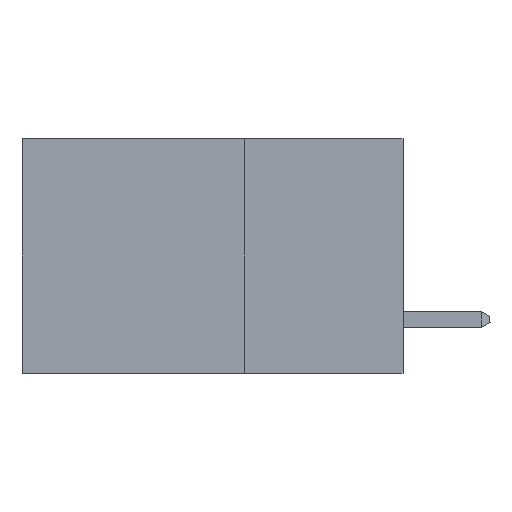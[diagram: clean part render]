
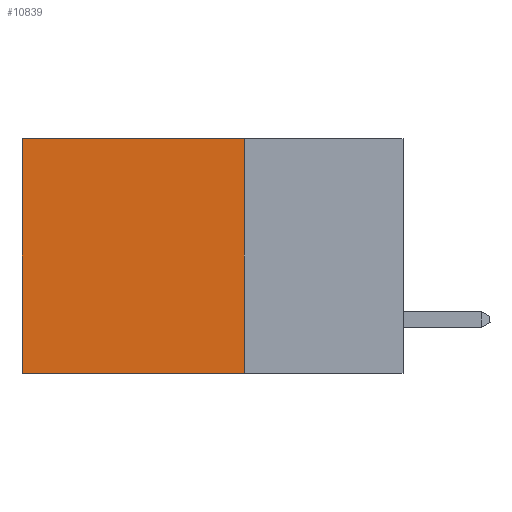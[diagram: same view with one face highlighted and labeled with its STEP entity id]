
A CAD part, left-side view. The second image highlights one B-rep face of the part: STEP entity #10839.
In plain terms, the highlighted planar face has unit normal (-1, 0, 0).
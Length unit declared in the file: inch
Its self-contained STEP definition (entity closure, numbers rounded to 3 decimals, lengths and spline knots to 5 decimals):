
#232 = CARTESIAN_POINT ( 'NONE',  ( 0.2875, 0.25, 0. ) ) ;
#489 = ORIENTED_EDGE ( 'NONE', *, *, #2428, .T. ) ;
#864 = VECTOR ( 'NONE', #17393, 39.37008 ) ;
#1470 = ORIENTED_EDGE ( 'NONE', *, *, #23373, .F. ) ;
#1630 = VERTEX_POINT ( 'NONE', #36720 ) ;
#2127 = VECTOR ( 'NONE', #3511, 39.37008 ) ;
#2197 = LINE ( 'NONE', #10476, #6208 ) ;
#2428 = EDGE_CURVE ( 'NONE', #10773, #30588, #11202, .T. ) ;
#2850 = DIRECTION ( 'NONE',  ( 0., 0., -1. ) ) ;
#3511 = DIRECTION ( 'NONE',  ( 0., 1., 0. ) ) ;
#6208 = VECTOR ( 'NONE', #19549, 39.37008 ) ;
#8319 = EDGE_CURVE ( 'NONE', #30588, #23445, #21845, .T. ) ;
#9410 = CARTESIAN_POINT ( 'NONE',  ( 0.2875, 0.6, -0.37 ) ) ;
#10476 = CARTESIAN_POINT ( 'NONE',  ( 0.2875, 0.25, 0. ) ) ;
#10515 = EDGE_LOOP ( 'NONE', ( #23994, #1470, #16117, #489 ) ) ;
#10773 = VERTEX_POINT ( 'NONE', #232 ) ;
#10839 = ADVANCED_FACE ( 'NONE', ( #13617 ), #36881, .F. ) ;
#11202 = LINE ( 'NONE', #35034, #864 ) ;
#13617 = FACE_OUTER_BOUND ( 'NONE', #10515, .T. ) ;
#16117 = ORIENTED_EDGE ( 'NONE', *, *, #21582, .F. ) ;
#17393 = DIRECTION ( 'NONE',  ( 0., 1., 0. ) ) ;
#18288 = CARTESIAN_POINT ( 'NONE',  ( 0.2875, 0.6, 0. ) ) ;
#19463 = CARTESIAN_POINT ( 'NONE',  ( 0.2875, 0.6, 0. ) ) ;
#19549 = DIRECTION ( 'NONE',  ( 0., 0., -1. ) ) ;
#21582 = EDGE_CURVE ( 'NONE', #10773, #1630, #2197, .T. ) ;
#21845 = LINE ( 'NONE', #19463, #24128 ) ;
#21852 = AXIS2_PLACEMENT_3D ( 'NONE', #31294, #37135, #2850 ) ;
#23373 = EDGE_CURVE ( 'NONE', #1630, #23445, #25505, .T. ) ;
#23445 = VERTEX_POINT ( 'NONE', #9410 ) ;
#23994 = ORIENTED_EDGE ( 'NONE', *, *, #8319, .T. ) ;
#24128 = VECTOR ( 'NONE', #36541, 39.37008 ) ;
#25505 = LINE ( 'NONE', #29323, #2127 ) ;
#29323 = CARTESIAN_POINT ( 'NONE',  ( 0.2875, 0.25, -0.37 ) ) ;
#30588 = VERTEX_POINT ( 'NONE', #18288 ) ;
#31294 = CARTESIAN_POINT ( 'NONE',  ( 0.2875, 0.25, 0. ) ) ;
#35034 = CARTESIAN_POINT ( 'NONE',  ( 0.2875, 0.25, 0. ) ) ;
#36541 = DIRECTION ( 'NONE',  ( 0., 0., -1. ) ) ;
#36720 = CARTESIAN_POINT ( 'NONE',  ( 0.2875, 0.25, -0.37 ) ) ;
#36881 = PLANE ( 'NONE',  #21852 ) ;
#37135 = DIRECTION ( 'NONE',  ( 1., 0., 0. ) ) ;
